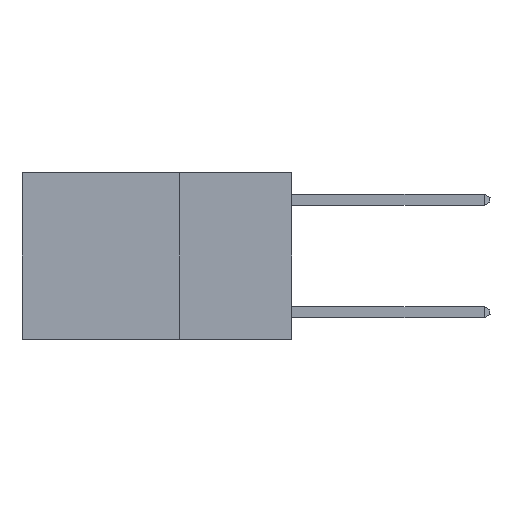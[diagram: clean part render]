
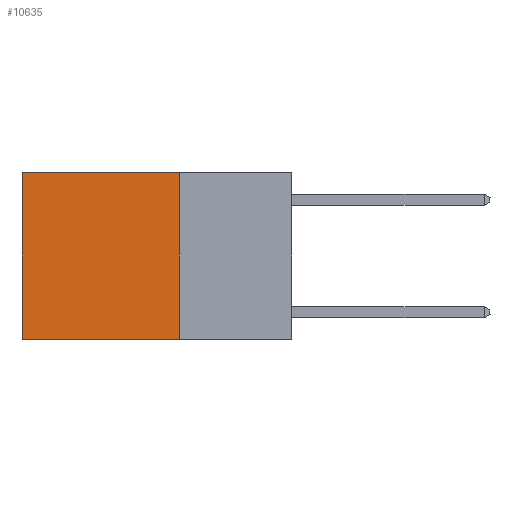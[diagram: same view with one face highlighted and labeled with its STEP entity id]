
A CAD part, left-side view. The second image highlights one B-rep face of the part: STEP entity #10635.
In plain terms, the highlighted planar face has unit normal (-1, 0, 0).
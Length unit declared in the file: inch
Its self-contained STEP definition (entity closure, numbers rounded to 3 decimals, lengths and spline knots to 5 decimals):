
#675 = LINE ( 'NONE', #5997, #5960 ) ;
#735 = ORIENTED_EDGE ( 'NONE', *, *, #11642, .F. ) ;
#1362 = CARTESIAN_POINT ( 'NONE',  ( 0.2625, 0.25, 0. ) ) ;
#1981 = ORIENTED_EDGE ( 'NONE', *, *, #6655, .T. ) ;
#2220 = DIRECTION ( 'NONE',  ( 0., 1., 0. ) ) ;
#2448 = CARTESIAN_POINT ( 'NONE',  ( 0.2625, 0.25, 0. ) ) ;
#2476 = VECTOR ( 'NONE', #2220, 39.37008 ) ;
#2747 = CARTESIAN_POINT ( 'NONE',  ( 0.2625, 0.25, -0.37 ) ) ;
#3294 = VECTOR ( 'NONE', #9649, 39.37008 ) ;
#3305 = ORIENTED_EDGE ( 'NONE', *, *, #8733, .F. ) ;
#4768 = CARTESIAN_POINT ( 'NONE',  ( 0.2625, 0.6, -0.37 ) ) ;
#5697 = ORIENTED_EDGE ( 'NONE', *, *, #12332, .T. ) ;
#5780 = LINE ( 'NONE', #1362, #6774 ) ;
#5960 = VECTOR ( 'NONE', #7005, 39.37008 ) ;
#5997 = CARTESIAN_POINT ( 'NONE',  ( 0.2625, 0.6, 0. ) ) ;
#6085 = VERTEX_POINT ( 'NONE', #7854 ) ;
#6655 = EDGE_CURVE ( 'NONE', #6085, #8140, #675, .T. ) ;
#6774 = VECTOR ( 'NONE', #10089, 39.37008 ) ;
#7005 = DIRECTION ( 'NONE',  ( 0., 0., -1. ) ) ;
#7121 = CARTESIAN_POINT ( 'NONE',  ( 0.2625, 0.25, 0. ) ) ;
#7670 = FACE_OUTER_BOUND ( 'NONE', #10947, .T. ) ;
#7848 = VERTEX_POINT ( 'NONE', #13627 ) ;
#7854 = CARTESIAN_POINT ( 'NONE',  ( 0.2625, 0.6, 0. ) ) ;
#8140 = VERTEX_POINT ( 'NONE', #4768 ) ;
#8700 = LINE ( 'NONE', #12979, #2476 ) ;
#8733 = EDGE_CURVE ( 'NONE', #7848, #8140, #12545, .T. ) ;
#9649 = DIRECTION ( 'NONE',  ( 0., 1., 0. ) ) ;
#10089 = DIRECTION ( 'NONE',  ( 0., 0., -1. ) ) ;
#10635 = ADVANCED_FACE ( 'NONE', ( #7670 ), #12098, .F. ) ;
#10947 = EDGE_LOOP ( 'NONE', ( #1981, #3305, #735, #5697 ) ) ;
#11208 = AXIS2_PLACEMENT_3D ( 'NONE', #2448, #12923, #13121 ) ;
#11642 = EDGE_CURVE ( 'NONE', #11726, #7848, #5780, .T. ) ;
#11726 = VERTEX_POINT ( 'NONE', #7121 ) ;
#12098 = PLANE ( 'NONE',  #11208 ) ;
#12332 = EDGE_CURVE ( 'NONE', #11726, #6085, #8700, .T. ) ;
#12545 = LINE ( 'NONE', #2747, #3294 ) ;
#12923 = DIRECTION ( 'NONE',  ( 1., 0., 0. ) ) ;
#12979 = CARTESIAN_POINT ( 'NONE',  ( 0.2625, 0.25, 0. ) ) ;
#13121 = DIRECTION ( 'NONE',  ( 0., 0., -1. ) ) ;
#13627 = CARTESIAN_POINT ( 'NONE',  ( 0.2625, 0.25, -0.37 ) ) ;
